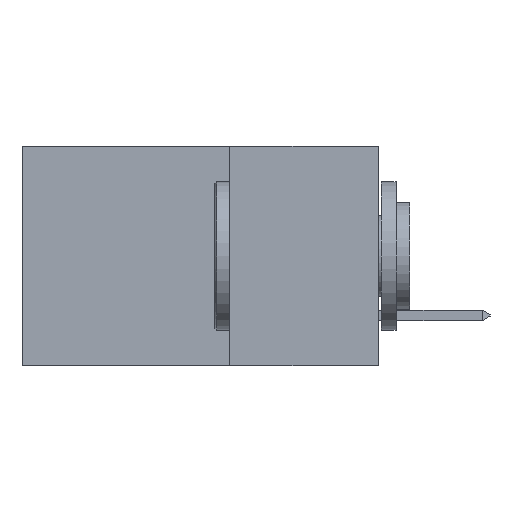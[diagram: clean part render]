
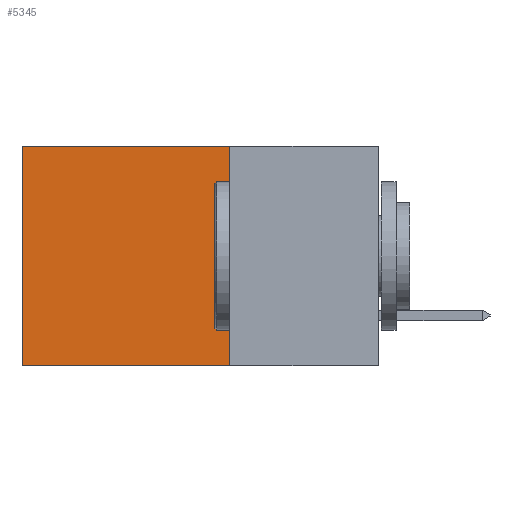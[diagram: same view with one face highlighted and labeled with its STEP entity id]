
A CAD part, left-side view. The second image highlights one B-rep face of the part: STEP entity #5345.
In plain terms, the highlighted planar face has unit normal (-1, 0, 0).
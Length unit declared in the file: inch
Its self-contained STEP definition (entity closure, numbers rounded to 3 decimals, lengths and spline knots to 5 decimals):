
#945 = CARTESIAN_POINT ( 'NONE',  ( 0.298, 0.25, 0. ) ) ;
#961 = VECTOR ( 'NONE', #9938, 39.37008 ) ;
#1523 = VERTEX_POINT ( 'NONE', #4025 ) ;
#1850 = DIRECTION ( 'NONE',  ( 0., 1., 0. ) ) ;
#2277 = VECTOR ( 'NONE', #3491, 39.37008 ) ;
#2305 = VECTOR ( 'NONE', #4397, 39.37008 ) ;
#2404 = ORIENTED_EDGE ( 'NONE', *, *, #6682, .T. ) ;
#2761 = VERTEX_POINT ( 'NONE', #4163 ) ;
#3351 = CARTESIAN_POINT ( 'NONE',  ( 0.298, 0.25, 0. ) ) ;
#3460 = EDGE_CURVE ( 'NONE', #10755, #6000, #8861, .T. ) ;
#3491 = DIRECTION ( 'NONE',  ( 0., 0., -1. ) ) ;
#3551 = CARTESIAN_POINT ( 'NONE',  ( 0.298, 0.25, -0.37 ) ) ;
#3874 = ORIENTED_EDGE ( 'NONE', *, *, #9192, .F. ) ;
#4025 = CARTESIAN_POINT ( 'NONE',  ( 0.298, 0.6, -0.37 ) ) ;
#4034 = ORIENTED_EDGE ( 'NONE', *, *, #3460, .F. ) ;
#4163 = CARTESIAN_POINT ( 'NONE',  ( 0.298, 0.6, 0. ) ) ;
#4397 = DIRECTION ( 'NONE',  ( 0., 1., 0. ) ) ;
#5043 = EDGE_LOOP ( 'NONE', ( #2404, #3874, #4034, #7158 ) ) ;
#5345 = ADVANCED_FACE ( 'NONE', ( #10110 ), #7480, .F. ) ;
#6000 = VERTEX_POINT ( 'NONE', #9085 ) ;
#6399 = VECTOR ( 'NONE', #1850, 39.37008 ) ;
#6682 = EDGE_CURVE ( 'NONE', #2761, #1523, #10087, .T. ) ;
#6975 = EDGE_CURVE ( 'NONE', #10755, #2761, #10842, .T. ) ;
#7156 = LINE ( 'NONE', #3551, #2305 ) ;
#7158 = ORIENTED_EDGE ( 'NONE', *, *, #6975, .T. ) ;
#7480 = PLANE ( 'NONE',  #10156 ) ;
#8861 = LINE ( 'NONE', #3351, #2277 ) ;
#9085 = CARTESIAN_POINT ( 'NONE',  ( 0.298, 0.25, -0.37 ) ) ;
#9192 = EDGE_CURVE ( 'NONE', #6000, #1523, #7156, .T. ) ;
#9934 = CARTESIAN_POINT ( 'NONE',  ( 0.298, 0.25, 0. ) ) ;
#9938 = DIRECTION ( 'NONE',  ( 0., 0., -1. ) ) ;
#10002 = CARTESIAN_POINT ( 'NONE',  ( 0.298, 0.25, 0. ) ) ;
#10087 = LINE ( 'NONE', #10741, #961 ) ;
#10110 = FACE_OUTER_BOUND ( 'NONE', #5043, .T. ) ;
#10156 = AXIS2_PLACEMENT_3D ( 'NONE', #10002, #10855, #10818 ) ;
#10741 = CARTESIAN_POINT ( 'NONE',  ( 0.298, 0.6, 0. ) ) ;
#10755 = VERTEX_POINT ( 'NONE', #9934 ) ;
#10818 = DIRECTION ( 'NONE',  ( 0., 0., -1. ) ) ;
#10842 = LINE ( 'NONE', #945, #6399 ) ;
#10855 = DIRECTION ( 'NONE',  ( 1., 0., 0. ) ) ;
